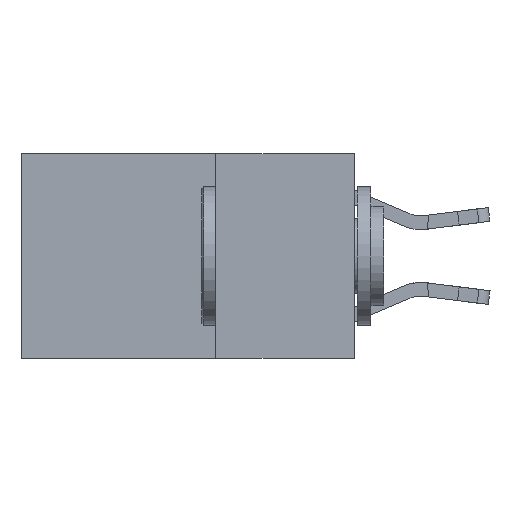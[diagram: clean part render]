
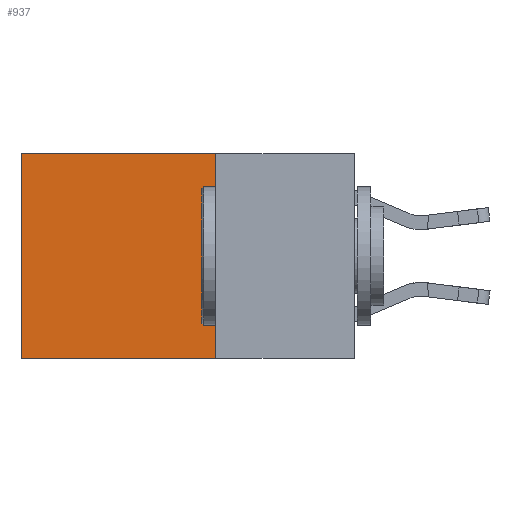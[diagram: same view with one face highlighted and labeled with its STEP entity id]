
A CAD part, left-side view. The second image highlights one B-rep face of the part: STEP entity #937.
In plain terms, the highlighted planar face has unit normal (-1, 0, 0).
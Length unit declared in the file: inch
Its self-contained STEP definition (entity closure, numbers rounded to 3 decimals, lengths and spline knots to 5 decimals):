
#29 = PLANE ( 'NONE',  #13738 ) ;
#573 = ORIENTED_EDGE ( 'NONE', *, *, #13188, .T. ) ;
#937 = ADVANCED_FACE ( 'NONE', ( #8437 ), #29, .F. ) ;
#1023 = DIRECTION ( 'NONE',  ( 0., 1., 0. ) ) ;
#1414 = VERTEX_POINT ( 'NONE', #21240 ) ;
#1958 = CARTESIAN_POINT ( 'NONE',  ( 0.2625, 0.6, 0. ) ) ;
#3361 = DIRECTION ( 'NONE',  ( 0., 0., -1. ) ) ;
#5403 = LINE ( 'NONE', #20080, #18336 ) ;
#5727 = VECTOR ( 'NONE', #1023, 39.37008 ) ;
#5747 = ORIENTED_EDGE ( 'NONE', *, *, #16136, .T. ) ;
#6141 = DIRECTION ( 'NONE',  ( 0., 1., 0. ) ) ;
#7692 = LINE ( 'NONE', #17944, #12154 ) ;
#8306 = DIRECTION ( 'NONE',  ( 0., 0., -1. ) ) ;
#8437 = FACE_OUTER_BOUND ( 'NONE', #14522, .T. ) ;
#10224 = ORIENTED_EDGE ( 'NONE', *, *, #18990, .F. ) ;
#10604 = CARTESIAN_POINT ( 'NONE',  ( 0.2625, 0.25, -0.37 ) ) ;
#11142 = ORIENTED_EDGE ( 'NONE', *, *, #20731, .F. ) ;
#11536 = CARTESIAN_POINT ( 'NONE',  ( 0.2625, 0.25, 0. ) ) ;
#11733 = CARTESIAN_POINT ( 'NONE',  ( 0.2625, 0.25, 0. ) ) ;
#12154 = VECTOR ( 'NONE', #6141, 39.37008 ) ;
#13188 = EDGE_CURVE ( 'NONE', #1414, #14110, #15910, .T. ) ;
#13448 = DIRECTION ( 'NONE',  ( 1., 0., 0. ) ) ;
#13713 = DIRECTION ( 'NONE',  ( 0., 0., -1. ) ) ;
#13738 = AXIS2_PLACEMENT_3D ( 'NONE', #11733, #13448, #3361 ) ;
#14110 = VERTEX_POINT ( 'NONE', #17878 ) ;
#14522 = EDGE_LOOP ( 'NONE', ( #573, #10224, #11142, #5747 ) ) ;
#15247 = VERTEX_POINT ( 'NONE', #10604 ) ;
#15910 = LINE ( 'NONE', #1958, #20354 ) ;
#16136 = EDGE_CURVE ( 'NONE', #17555, #1414, #7692, .T. ) ;
#17555 = VERTEX_POINT ( 'NONE', #11536 ) ;
#17878 = CARTESIAN_POINT ( 'NONE',  ( 0.2625, 0.6, -0.37 ) ) ;
#17944 = CARTESIAN_POINT ( 'NONE',  ( 0.2625, 0.25, 0. ) ) ;
#18336 = VECTOR ( 'NONE', #8306, 39.37008 ) ;
#18683 = LINE ( 'NONE', #20110, #5727 ) ;
#18990 = EDGE_CURVE ( 'NONE', #15247, #14110, #18683, .T. ) ;
#20080 = CARTESIAN_POINT ( 'NONE',  ( 0.2625, 0.25, 0. ) ) ;
#20110 = CARTESIAN_POINT ( 'NONE',  ( 0.2625, 0.25, -0.37 ) ) ;
#20354 = VECTOR ( 'NONE', #13713, 39.37008 ) ;
#20731 = EDGE_CURVE ( 'NONE', #17555, #15247, #5403, .T. ) ;
#21240 = CARTESIAN_POINT ( 'NONE',  ( 0.2625, 0.6, 0. ) ) ;
